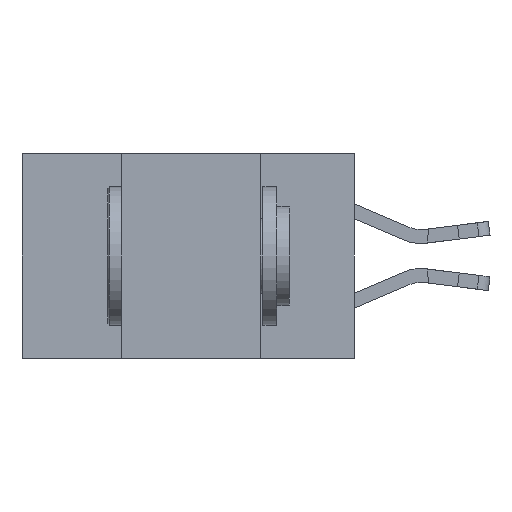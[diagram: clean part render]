
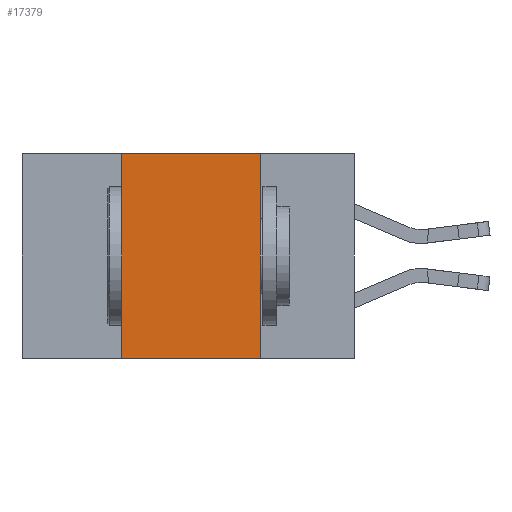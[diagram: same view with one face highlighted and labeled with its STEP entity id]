
A CAD part, left-side view. The second image highlights one B-rep face of the part: STEP entity #17379.
In plain terms, the highlighted planar face has unit normal (-1, 0, 0).
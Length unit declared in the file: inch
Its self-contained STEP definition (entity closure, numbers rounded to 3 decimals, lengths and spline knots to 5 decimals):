
#438 = LINE ( 'NONE', #10077, #11029 ) ;
#540 = CARTESIAN_POINT ( 'NONE',  ( 0., 0.6, 0. ) ) ;
#1379 = VERTEX_POINT ( 'NONE', #4079 ) ;
#1577 = VERTEX_POINT ( 'NONE', #9700 ) ;
#2274 = EDGE_CURVE ( 'NONE', #1379, #17317, #15986, .T. ) ;
#2852 = CARTESIAN_POINT ( 'NONE',  ( 0., 0.42, -0.37 ) ) ;
#3205 = EDGE_CURVE ( 'NONE', #8092, #1577, #12050, .T. ) ;
#4012 = CARTESIAN_POINT ( 'NONE',  ( 0., 0.6, -0.37 ) ) ;
#4019 = ORIENTED_EDGE ( 'NONE', *, *, #2274, .F. ) ;
#4079 = CARTESIAN_POINT ( 'NONE',  ( 0., 0.17, 0. ) ) ;
#4699 = VECTOR ( 'NONE', #5607, 39.37008 ) ;
#4998 = EDGE_LOOP ( 'NONE', ( #4019, #14486, #6886, #12849 ) ) ;
#5432 = DIRECTION ( 'NONE',  ( 0., -1., 0. ) ) ;
#5607 = DIRECTION ( 'NONE',  ( 0., 0., 1. ) ) ;
#5729 = CARTESIAN_POINT ( 'NONE',  ( 0., 0.42, 0. ) ) ;
#6094 = DIRECTION ( 'NONE',  ( 0., 0., -1. ) ) ;
#6636 = EDGE_CURVE ( 'NONE', #1577, #1379, #438, .T. ) ;
#6886 = ORIENTED_EDGE ( 'NONE', *, *, #3205, .F. ) ;
#8092 = VERTEX_POINT ( 'NONE', #2852 ) ;
#8459 = VECTOR ( 'NONE', #13176, 39.37008 ) ;
#9700 = CARTESIAN_POINT ( 'NONE',  ( 0., 0.42, 0. ) ) ;
#10077 = CARTESIAN_POINT ( 'NONE',  ( 0., 0.6, 0. ) ) ;
#10226 = PLANE ( 'NONE',  #14150 ) ;
#11029 = VECTOR ( 'NONE', #14398, 39.37008 ) ;
#11082 = VECTOR ( 'NONE', #5432, 39.37008 ) ;
#11497 = LINE ( 'NONE', #4012, #11082 ) ;
#12050 = LINE ( 'NONE', #5729, #4699 ) ;
#12740 = CARTESIAN_POINT ( 'NONE',  ( 0., 0.17, -0.37 ) ) ;
#12849 = ORIENTED_EDGE ( 'NONE', *, *, #15390, .T. ) ;
#13176 = DIRECTION ( 'NONE',  ( 0., 0., -1. ) ) ;
#14150 = AXIS2_PLACEMENT_3D ( 'NONE', #540, #14226, #6094 ) ;
#14226 = DIRECTION ( 'NONE',  ( 1., 0., 0. ) ) ;
#14398 = DIRECTION ( 'NONE',  ( 0., -1., 0. ) ) ;
#14486 = ORIENTED_EDGE ( 'NONE', *, *, #6636, .F. ) ;
#14896 = CARTESIAN_POINT ( 'NONE',  ( 0., 0.17, 0. ) ) ;
#15390 = EDGE_CURVE ( 'NONE', #8092, #17317, #11497, .T. ) ;
#15986 = LINE ( 'NONE', #14896, #8459 ) ;
#17183 = FACE_OUTER_BOUND ( 'NONE', #4998, .T. ) ;
#17317 = VERTEX_POINT ( 'NONE', #12740 ) ;
#17379 = ADVANCED_FACE ( 'NONE', ( #17183 ), #10226, .F. ) ;
